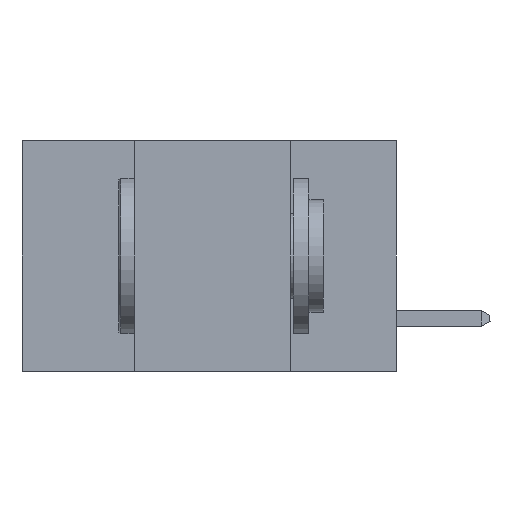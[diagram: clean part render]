
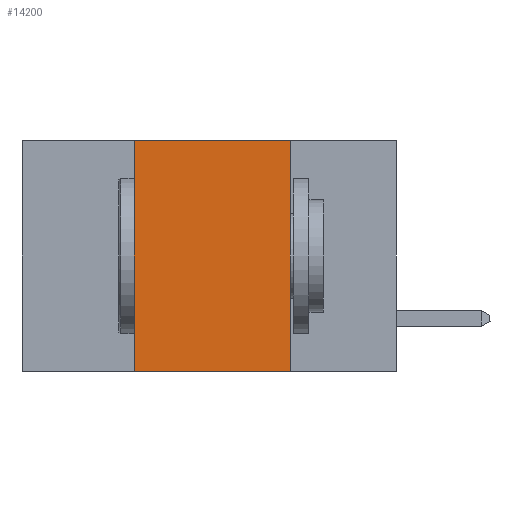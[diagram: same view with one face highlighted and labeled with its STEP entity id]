
A CAD part, left-side view. The second image highlights one B-rep face of the part: STEP entity #14200.
In plain terms, the highlighted planar face has unit normal (-1, 0, 0).
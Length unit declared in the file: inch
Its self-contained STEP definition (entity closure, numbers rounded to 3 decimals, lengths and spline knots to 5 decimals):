
#1703 = EDGE_CURVE ( 'NONE', #20751, #8776, #10397, .T. ) ;
#2996 = EDGE_CURVE ( 'NONE', #20751, #10331, #10674, .T. ) ;
#5998 = DIRECTION ( 'NONE',  ( 0., -1., 0. ) ) ;
#6750 = ORIENTED_EDGE ( 'NONE', *, *, #6846, .F. ) ;
#6846 = EDGE_CURVE ( 'NONE', #12837, #8776, #19962, .T. ) ;
#7291 = CARTESIAN_POINT ( 'NONE',  ( 0., 0.42, -0.37 ) ) ;
#7812 = CARTESIAN_POINT ( 'NONE',  ( 0., 0.6, -0.37 ) ) ;
#7871 = DIRECTION ( 'NONE',  ( 0., -1., 0. ) ) ;
#8776 = VERTEX_POINT ( 'NONE', #20541 ) ;
#9124 = EDGE_LOOP ( 'NONE', ( #6750, #12357, #21991, #12932 ) ) ;
#9130 = VECTOR ( 'NONE', #5998, 39.37008 ) ;
#10331 = VERTEX_POINT ( 'NONE', #22861 ) ;
#10397 = LINE ( 'NONE', #7812, #15426 ) ;
#10535 = DIRECTION ( 'NONE',  ( 0., 0., -1. ) ) ;
#10674 = LINE ( 'NONE', #15272, #11288 ) ;
#10675 = DIRECTION ( 'NONE',  ( 1., 0., 0. ) ) ;
#10908 = CARTESIAN_POINT ( 'NONE',  ( 0., 0.17, 0. ) ) ;
#11288 = VECTOR ( 'NONE', #15247, 39.37008 ) ;
#11806 = CARTESIAN_POINT ( 'NONE',  ( 0., 0.17, 0. ) ) ;
#12357 = ORIENTED_EDGE ( 'NONE', *, *, #18550, .F. ) ;
#12541 = CARTESIAN_POINT ( 'NONE',  ( 0., 0.6, 0. ) ) ;
#12837 = VERTEX_POINT ( 'NONE', #10908 ) ;
#12932 = ORIENTED_EDGE ( 'NONE', *, *, #1703, .T. ) ;
#14200 = ADVANCED_FACE ( 'NONE', ( #22184 ), #19851, .F. ) ;
#15247 = DIRECTION ( 'NONE',  ( 0., 0., 1. ) ) ;
#15272 = CARTESIAN_POINT ( 'NONE',  ( 0., 0.42, 0. ) ) ;
#15426 = VECTOR ( 'NONE', #7871, 39.37008 ) ;
#16301 = VECTOR ( 'NONE', #10535, 39.37008 ) ;
#18550 = EDGE_CURVE ( 'NONE', #10331, #12837, #18975, .T. ) ;
#18975 = LINE ( 'NONE', #18977, #9130 ) ;
#18977 = CARTESIAN_POINT ( 'NONE',  ( 0., 0.6, 0. ) ) ;
#19851 = PLANE ( 'NONE',  #21795 ) ;
#19962 = LINE ( 'NONE', #11806, #16301 ) ;
#20541 = CARTESIAN_POINT ( 'NONE',  ( 0., 0.17, -0.37 ) ) ;
#20751 = VERTEX_POINT ( 'NONE', #7291 ) ;
#21795 = AXIS2_PLACEMENT_3D ( 'NONE', #12541, #10675, #23417 ) ;
#21991 = ORIENTED_EDGE ( 'NONE', *, *, #2996, .F. ) ;
#22184 = FACE_OUTER_BOUND ( 'NONE', #9124, .T. ) ;
#22861 = CARTESIAN_POINT ( 'NONE',  ( 0., 0.42, 0. ) ) ;
#23417 = DIRECTION ( 'NONE',  ( 0., 0., -1. ) ) ;
